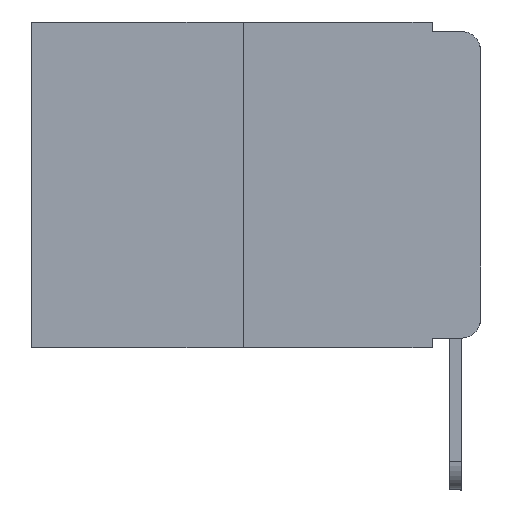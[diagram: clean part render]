
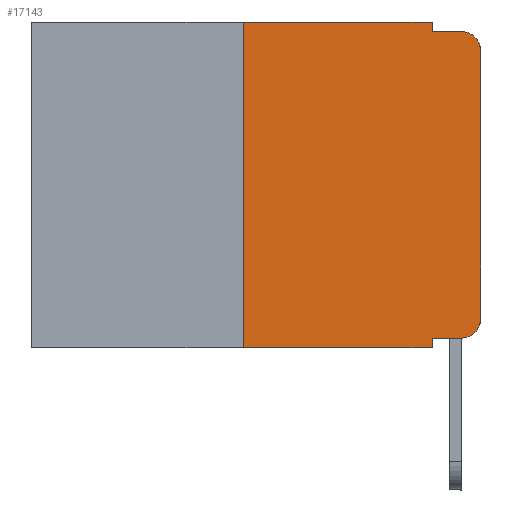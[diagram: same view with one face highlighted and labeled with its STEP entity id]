
A CAD part, left-side view. The second image highlights one B-rep face of the part: STEP entity #17143.
In plain terms, the highlighted planar face has unit normal (-1, 0, 0).
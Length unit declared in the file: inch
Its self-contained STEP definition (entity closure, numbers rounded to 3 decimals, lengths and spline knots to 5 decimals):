
#256 = CARTESIAN_POINT ( 'NONE',  ( 0., 0.051, -0.01 ) ) ;
#327 = VECTOR ( 'NONE', #758, 39.37008 ) ;
#347 = CARTESIAN_POINT ( 'NONE',  ( 0., 0.051, -0.01 ) ) ;
#374 = DIRECTION ( 'NONE',  ( 0., 0., -1. ) ) ;
#422 = DIRECTION ( 'NONE',  ( -1., 0., 0. ) ) ;
#515 = AXIS2_PLACEMENT_3D ( 'NONE', #11303, #3694, #11218 ) ;
#636 = VERTEX_POINT ( 'NONE', #12373 ) ;
#725 = PLANE ( 'NONE',  #515 ) ;
#758 = DIRECTION ( 'NONE',  ( 0., 0., 1. ) ) ;
#801 = EDGE_CURVE ( 'NONE', #8675, #16614, #14168, .T. ) ;
#1212 = ORIENTED_EDGE ( 'NONE', *, *, #2703, .T. ) ;
#1649 = LINE ( 'NONE', #256, #5220 ) ;
#1739 = LINE ( 'NONE', #4803, #12015 ) ;
#1781 = CARTESIAN_POINT ( 'NONE',  ( 0., 0.25, 0. ) ) ;
#1955 = CARTESIAN_POINT ( 'NONE',  ( 0., 0., 0. ) ) ;
#2047 = EDGE_CURVE ( 'NONE', #4035, #7936, #7304, .T. ) ;
#2203 = FACE_OUTER_BOUND ( 'NONE', #6703, .T. ) ;
#2274 = CARTESIAN_POINT ( 'NONE',  ( 0., 0.051, 0. ) ) ;
#2538 = VERTEX_POINT ( 'NONE', #4045 ) ;
#2667 = CARTESIAN_POINT ( 'NONE',  ( 0., 0.051, -0.333 ) ) ;
#2703 = EDGE_CURVE ( 'NONE', #2538, #636, #3783, .T. ) ;
#2764 = ORIENTED_EDGE ( 'NONE', *, *, #2047, .F. ) ;
#2768 = CARTESIAN_POINT ( 'NONE',  ( 0., 0.02, -0.333 ) ) ;
#3110 = LINE ( 'NONE', #1955, #10194 ) ;
#3285 = DIRECTION ( 'NONE',  ( 0., -1., 0. ) ) ;
#3498 = VERTEX_POINT ( 'NONE', #14365 ) ;
#3694 = DIRECTION ( 'NONE',  ( 1., 0., 0. ) ) ;
#3783 = CIRCLE ( 'NONE', #6007, 0.02 ) ;
#4035 = VERTEX_POINT ( 'NONE', #2274 ) ;
#4045 = CARTESIAN_POINT ( 'NONE',  ( 0., 0., -0.03 ) ) ;
#4054 = ORIENTED_EDGE ( 'NONE', *, *, #4300, .T. ) ;
#4300 = EDGE_CURVE ( 'NONE', #4475, #11441, #4659, .T. ) ;
#4475 = VERTEX_POINT ( 'NONE', #2768 ) ;
#4659 = CIRCLE ( 'NONE', #8513, 0.02 ) ;
#4803 = CARTESIAN_POINT ( 'NONE',  ( 0., 0.473, -0.343 ) ) ;
#5002 = ORIENTED_EDGE ( 'NONE', *, *, #9606, .F. ) ;
#5220 = VECTOR ( 'NONE', #11010, 39.37008 ) ;
#5535 = DIRECTION ( 'NONE',  ( -1., 0., 0. ) ) ;
#5571 = CARTESIAN_POINT ( 'NONE',  ( 0., 0.051, 0. ) ) ;
#5701 = ORIENTED_EDGE ( 'NONE', *, *, #12649, .T. ) ;
#5783 = CARTESIAN_POINT ( 'NONE',  ( 0., 0.473, 0. ) ) ;
#6007 = AXIS2_PLACEMENT_3D ( 'NONE', #16312, #5535, #374 ) ;
#6703 = EDGE_LOOP ( 'NONE', ( #7624, #1212, #12091, #2764, #9627, #14947, #5701, #5002, #8714, #4054 ) ) ;
#6897 = DIRECTION ( 'NONE',  ( 0., -1., 0. ) ) ;
#6951 = EDGE_CURVE ( 'NONE', #16614, #4035, #8434, .T. ) ;
#7205 = DIRECTION ( 'NONE',  ( 0., 0., -1. ) ) ;
#7275 = LINE ( 'NONE', #15137, #16876 ) ;
#7304 = LINE ( 'NONE', #9969, #7869 ) ;
#7624 = ORIENTED_EDGE ( 'NONE', *, *, #16582, .T. ) ;
#7869 = VECTOR ( 'NONE', #15169, 39.37008 ) ;
#7936 = VERTEX_POINT ( 'NONE', #347 ) ;
#8434 = LINE ( 'NONE', #5783, #9426 ) ;
#8513 = AXIS2_PLACEMENT_3D ( 'NONE', #12390, #422, #7205 ) ;
#8675 = VERTEX_POINT ( 'NONE', #14660 ) ;
#8714 = ORIENTED_EDGE ( 'NONE', *, *, #9796, .T. ) ;
#9426 = VECTOR ( 'NONE', #6897, 39.37008 ) ;
#9606 = EDGE_CURVE ( 'NONE', #10004, #3498, #16074, .T. ) ;
#9627 = ORIENTED_EDGE ( 'NONE', *, *, #6951, .F. ) ;
#9796 = EDGE_CURVE ( 'NONE', #10004, #4475, #7275, .T. ) ;
#9969 = CARTESIAN_POINT ( 'NONE',  ( 0., 0.051, 0. ) ) ;
#10004 = VERTEX_POINT ( 'NONE', #2667 ) ;
#10194 = VECTOR ( 'NONE', #13653, 39.37008 ) ;
#11010 = DIRECTION ( 'NONE',  ( 0., -1., 0. ) ) ;
#11218 = DIRECTION ( 'NONE',  ( 0., 0., -1. ) ) ;
#11303 = CARTESIAN_POINT ( 'NONE',  ( 0., 0.473, 0. ) ) ;
#11441 = VERTEX_POINT ( 'NONE', #13900 ) ;
#12015 = VECTOR ( 'NONE', #16556, 39.37008 ) ;
#12091 = ORIENTED_EDGE ( 'NONE', *, *, #15564, .F. ) ;
#12373 = CARTESIAN_POINT ( 'NONE',  ( 0., 0.02, -0.01 ) ) ;
#12390 = CARTESIAN_POINT ( 'NONE',  ( 0., 0.02, -0.313 ) ) ;
#12649 = EDGE_CURVE ( 'NONE', #8675, #3498, #1739, .T. ) ;
#12801 = CARTESIAN_POINT ( 'NONE',  ( 0., 0.25, 0. ) ) ;
#13653 = DIRECTION ( 'NONE',  ( 0., 0., 1. ) ) ;
#13900 = CARTESIAN_POINT ( 'NONE',  ( 0., 0., -0.313 ) ) ;
#14168 = LINE ( 'NONE', #12801, #327 ) ;
#14365 = CARTESIAN_POINT ( 'NONE',  ( 0., 0.051, -0.343 ) ) ;
#14660 = CARTESIAN_POINT ( 'NONE',  ( 0., 0.25, -0.343 ) ) ;
#14793 = DIRECTION ( 'NONE',  ( 0., 0., -1. ) ) ;
#14947 = ORIENTED_EDGE ( 'NONE', *, *, #801, .F. ) ;
#15137 = CARTESIAN_POINT ( 'NONE',  ( 0., 0.051, -0.333 ) ) ;
#15169 = DIRECTION ( 'NONE',  ( 0., 0., -1. ) ) ;
#15496 = VECTOR ( 'NONE', #14793, 39.37008 ) ;
#15564 = EDGE_CURVE ( 'NONE', #7936, #636, #1649, .T. ) ;
#16074 = LINE ( 'NONE', #5571, #15496 ) ;
#16312 = CARTESIAN_POINT ( 'NONE',  ( 0., 0.02, -0.03 ) ) ;
#16556 = DIRECTION ( 'NONE',  ( 0., -1., 0. ) ) ;
#16582 = EDGE_CURVE ( 'NONE', #11441, #2538, #3110, .T. ) ;
#16614 = VERTEX_POINT ( 'NONE', #1781 ) ;
#16876 = VECTOR ( 'NONE', #3285, 39.37008 ) ;
#17143 = ADVANCED_FACE ( 'NONE', ( #2203 ), #725, .F. ) ;
